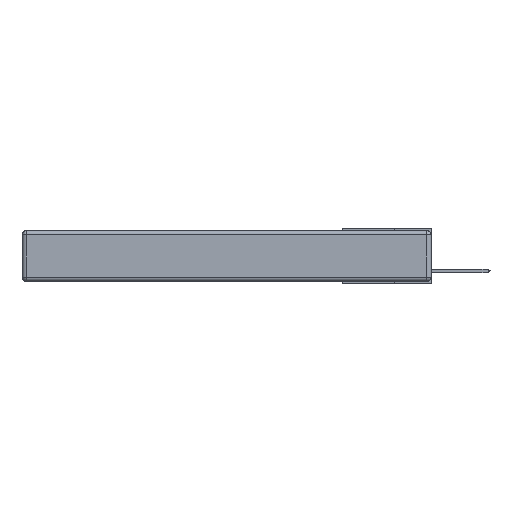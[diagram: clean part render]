
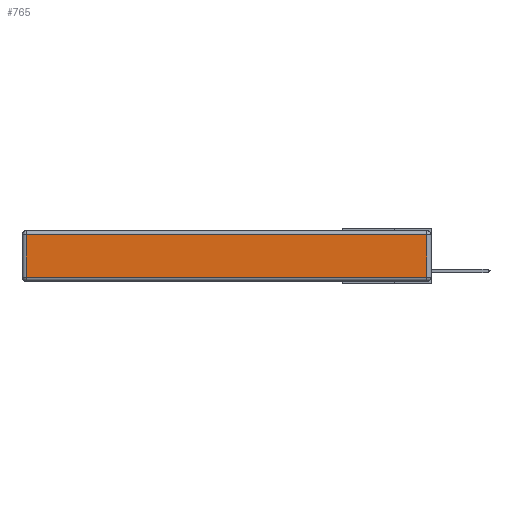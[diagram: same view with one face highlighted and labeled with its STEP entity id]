
A CAD part, left-side view. The second image highlights one B-rep face of the part: STEP entity #765.
In plain terms, the highlighted planar face has unit normal (-1, 0, 0).
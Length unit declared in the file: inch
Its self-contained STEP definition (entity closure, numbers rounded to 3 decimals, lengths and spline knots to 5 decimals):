
#456 = DIRECTION ( 'NONE',  ( 0., 0., 1. ) ) ;
#521 = CARTESIAN_POINT ( 'NONE',  ( 0., 0.03, -0.343 ) ) ;
#670 = AXIS2_PLACEMENT_3D ( 'NONE', #7053, #13631, #18466 ) ;
#765 = ADVANCED_FACE ( 'NONE', ( #9809 ), #18400, .T. ) ;
#807 = CARTESIAN_POINT ( 'NONE',  ( 0., 2.72, -0.03 ) ) ;
#1071 = DIRECTION ( 'NONE',  ( 0., 0., -1. ) ) ;
#1945 = DIRECTION ( 'NONE',  ( 0., -1., 0. ) ) ;
#2906 = EDGE_CURVE ( 'NONE', #10968, #21001, #13058, .T. ) ;
#3236 = LINE ( 'NONE', #8424, #6556 ) ;
#5389 = EDGE_CURVE ( 'NONE', #7234, #10968, #3236, .T. ) ;
#6556 = VECTOR ( 'NONE', #1945, 39.37008 ) ;
#7053 = CARTESIAN_POINT ( 'NONE',  ( 0., 0., -0.343 ) ) ;
#7234 = VERTEX_POINT ( 'NONE', #15731 ) ;
#7441 = ORIENTED_EDGE ( 'NONE', *, *, #2906, .T. ) ;
#8245 = EDGE_LOOP ( 'NONE', ( #9059, #7441, #19707, #15006 ) ) ;
#8424 = CARTESIAN_POINT ( 'NONE',  ( 0., 0., -0.313 ) ) ;
#8729 = VECTOR ( 'NONE', #456, 39.37008 ) ;
#9059 = ORIENTED_EDGE ( 'NONE', *, *, #5389, .T. ) ;
#9666 = DIRECTION ( 'NONE',  ( 0., 1., 0. ) ) ;
#9809 = FACE_OUTER_BOUND ( 'NONE', #8245, .T. ) ;
#10540 = LINE ( 'NONE', #15467, #12582 ) ;
#10968 = VERTEX_POINT ( 'NONE', #14337 ) ;
#11454 = CARTESIAN_POINT ( 'NONE',  ( 0., 2.75, -0.03 ) ) ;
#12582 = VECTOR ( 'NONE', #1071, 39.37008 ) ;
#13058 = LINE ( 'NONE', #521, #8729 ) ;
#13369 = EDGE_CURVE ( 'NONE', #20197, #7234, #10540, .T. ) ;
#13631 = DIRECTION ( 'NONE',  ( -1., 0., 0. ) ) ;
#14337 = CARTESIAN_POINT ( 'NONE',  ( 0., 0.03, -0.313 ) ) ;
#15006 = ORIENTED_EDGE ( 'NONE', *, *, #13369, .T. ) ;
#15466 = LINE ( 'NONE', #11454, #19299 ) ;
#15467 = CARTESIAN_POINT ( 'NONE',  ( 0., 2.72, -0.343 ) ) ;
#15731 = CARTESIAN_POINT ( 'NONE',  ( 0., 2.72, -0.313 ) ) ;
#18025 = EDGE_CURVE ( 'NONE', #21001, #20197, #15466, .T. ) ;
#18400 = PLANE ( 'NONE',  #670 ) ;
#18466 = DIRECTION ( 'NONE',  ( 0., 0., 1. ) ) ;
#19299 = VECTOR ( 'NONE', #9666, 39.37008 ) ;
#19707 = ORIENTED_EDGE ( 'NONE', *, *, #18025, .T. ) ;
#20197 = VERTEX_POINT ( 'NONE', #807 ) ;
#20423 = CARTESIAN_POINT ( 'NONE',  ( 0., 0.03, -0.03 ) ) ;
#21001 = VERTEX_POINT ( 'NONE', #20423 ) ;
